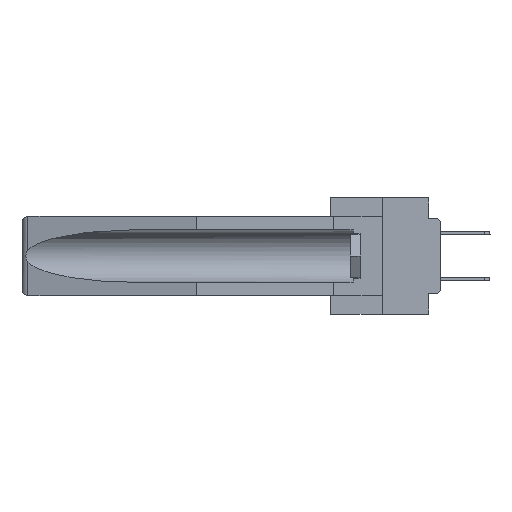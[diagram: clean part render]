
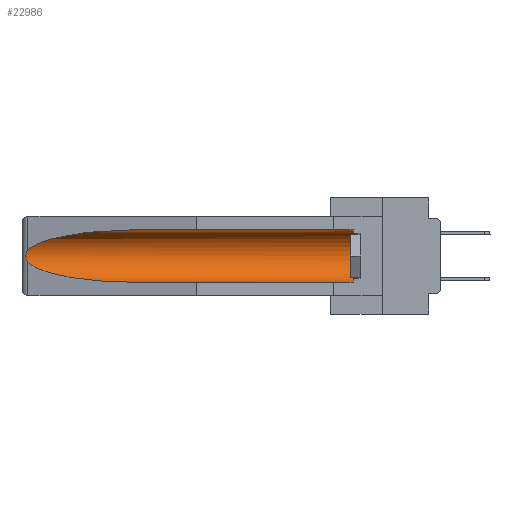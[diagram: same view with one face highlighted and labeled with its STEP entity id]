
A CAD part, left-side view. The second image highlights one B-rep face of the part: STEP entity #22986.
In plain terms, the highlighted cylindrical face has radius 2.857 mm (diameter 5.715 mm), a partial arc.
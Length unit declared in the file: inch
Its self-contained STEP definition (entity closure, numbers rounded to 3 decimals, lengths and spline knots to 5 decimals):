
#192 = CARTESIAN_POINT ( 'NONE',  ( 0.25451, 1.48313, -0.09465 ) ) ;
#2020 = FACE_OUTER_BOUND ( 'NONE', #16455, .T. ) ;
#2056 = ORIENTED_EDGE ( 'NONE', *, *, #12006, .T. ) ;
#2120 = CARTESIAN_POINT ( 'NONE',  ( 0.26537, 1.52718, -0.19328 ) ) ;
#2142 = CARTESIAN_POINT ( 'NONE',  ( 0.155, 1.07973, -0.284 ) ) ;
#2314 = CARTESIAN_POINT ( 'NONE',  ( 0.26537, 1.52718, -0.19328 ) ) ;
#2324 = CARTESIAN_POINT ( 'NONE',  ( 0.2673, 1.53269, -0.17917 ) ) ;
#2793 = EDGE_CURVE ( 'NONE', #16235, #20922, #7235, .T. ) ;
#2963 = EDGE_CURVE ( 'NONE', #4122, #29052, #12959, .T. ) ;
#3872 = CARTESIAN_POINT ( 'NONE',  ( 0.155, 1.07973, -0.059 ) ) ;
#4122 = VERTEX_POINT ( 'NONE', #9852 ) ;
#4868 = LINE ( 'NONE', #5699, #19625 ) ;
#5378 =( BOUNDED_CURVE ( )  B_SPLINE_CURVE ( 3, ( #25548, #13990, #192, #20624 ),
 .UNSPECIFIED., .F., .F. ) 
 B_SPLINE_CURVE_WITH_KNOTS ( ( 4, 4 ),
 ( 4.71239, 6.08839 ),
 .UNSPECIFIED. ) 
 CURVE ( )  GEOMETRIC_REPRESENTATION_ITEM ( )  RATIONAL_B_SPLINE_CURVE ( ( 1., 0.848, 0.848, 1. ) ) 
 REPRESENTATION_ITEM ( '' )  );
#5699 = CARTESIAN_POINT ( 'NONE',  ( 0.155, -0.30754, -0.284 ) ) ;
#5788 = VECTOR ( 'NONE', #6895, 39.37008 ) ;
#6256 = CARTESIAN_POINT ( 'NONE',  ( 0.26654, 1.53092, -0.15636 ) ) ;
#6895 = DIRECTION ( 'NONE',  ( 0., 1., 0. ) ) ;
#7235 =( BOUNDED_CURVE ( )  B_SPLINE_CURVE ( 3, ( #11639, #7424, #16296, #18592 ),
 .UNSPECIFIED., .F., .F. ) 
 B_SPLINE_CURVE_WITH_KNOTS ( ( 4, 4 ),
 ( 0.1948, 1.5708 ),
 .UNSPECIFIED. ) 
 CURVE ( )  GEOMETRIC_REPRESENTATION_ITEM ( )  RATIONAL_B_SPLINE_CURVE ( ( 1., 0.848, 0.848, 1. ) ) 
 REPRESENTATION_ITEM ( '' )  );
#7424 = CARTESIAN_POINT ( 'NONE',  ( 0.25451, 1.48313, -0.24835 ) ) ;
#8125 = CYLINDRICAL_SURFACE ( 'NONE', #21301, 0.1125 ) ;
#8450 = CARTESIAN_POINT ( 'NONE',  ( 0.26597, 1.52961, -0.15275 ) ) ;
#9852 = CARTESIAN_POINT ( 'NONE',  ( 0.155, 0.126, -0.059 ) ) ;
#10195 = DIRECTION ( 'NONE',  ( 0., 0., 1. ) ) ;
#10213 = DIRECTION ( 'NONE',  ( 0., 1., 0. ) ) ;
#10776 = CARTESIAN_POINT ( 'NONE',  ( 0.2675, 1.53308, -0.16763 ) ) ;
#11327 = VERTEX_POINT ( 'NONE', #21491 ) ;
#11628 = ORIENTED_EDGE ( 'NONE', *, *, #15197, .F. ) ;
#11639 = CARTESIAN_POINT ( 'NONE',  ( 0.26537, 1.52718, -0.19328 ) ) ;
#11834 = CARTESIAN_POINT ( 'NONE',  ( 0.155, -0.30754, -0.1715 ) ) ;
#12006 = EDGE_CURVE ( 'NONE', #11327, #4122, #24138, .T. ) ;
#12363 = EDGE_CURVE ( 'NONE', #29052, #29511, #5378, .T. ) ;
#12959 = LINE ( 'NONE', #14118, #5788 ) ;
#13074 = CARTESIAN_POINT ( 'NONE',  ( 0.2675, 1.53308, -0.17534 ) ) ;
#13815 = CARTESIAN_POINT ( 'NONE',  ( 0.26537, 1.52718, -0.14972 ) ) ;
#13990 = CARTESIAN_POINT ( 'NONE',  ( 0.21114, 1.30732, -0.059 ) ) ;
#14118 = CARTESIAN_POINT ( 'NONE',  ( 0.155, -0.30754, -0.059 ) ) ;
#14432 = B_SPLINE_CURVE_WITH_KNOTS ( 'NONE', 3,
 ( #18319, #8450, #6256, #24533, #10776, #13074, #2324, #29193, #15297, #2120 ),
 .UNSPECIFIED., .F., .F.,
 ( 4, 2, 2, 2, 4 ),
 ( 0., 0.00029, 0.00058, 0.00087, 0.00117 ),
 .UNSPECIFIED. ) ;
#15197 = EDGE_CURVE ( 'NONE', #11327, #20922, #4868, .T. ) ;
#15297 = CARTESIAN_POINT ( 'NONE',  ( 0.26597, 1.5296, -0.19026 ) ) ;
#16235 = VERTEX_POINT ( 'NONE', #2314 ) ;
#16296 = CARTESIAN_POINT ( 'NONE',  ( 0.21114, 1.30732, -0.284 ) ) ;
#16455 = EDGE_LOOP ( 'NONE', ( #20876, #25119, #20142, #11628, #2056, #27660 ) ) ;
#18319 = CARTESIAN_POINT ( 'NONE',  ( 0.26537, 1.52718, -0.14972 ) ) ;
#18592 = CARTESIAN_POINT ( 'NONE',  ( 0.155, 1.07973, -0.284 ) ) ;
#19348 = CARTESIAN_POINT ( 'NONE',  ( 0.155, 0.126, -0.1715 ) ) ;
#19625 = VECTOR ( 'NONE', #10213, 39.37008 ) ;
#20142 = ORIENTED_EDGE ( 'NONE', *, *, #2793, .T. ) ;
#20624 = CARTESIAN_POINT ( 'NONE',  ( 0.26537, 1.52718, -0.14972 ) ) ;
#20876 = ORIENTED_EDGE ( 'NONE', *, *, #12363, .T. ) ;
#20922 = VERTEX_POINT ( 'NONE', #2142 ) ;
#21301 = AXIS2_PLACEMENT_3D ( 'NONE', #11834, #25324, #23384 ) ;
#21491 = CARTESIAN_POINT ( 'NONE',  ( 0.155, 0.126, -0.284 ) ) ;
#22986 = ADVANCED_FACE ( 'NONE', ( #2020 ), #8125, .F. ) ;
#23384 = DIRECTION ( 'NONE',  ( 0., 0., 1. ) ) ;
#24138 = CIRCLE ( 'NONE', #27842, 0.1125 ) ;
#24533 = CARTESIAN_POINT ( 'NONE',  ( 0.2673, 1.5327, -0.16383 ) ) ;
#25119 = ORIENTED_EDGE ( 'NONE', *, *, #25234, .T. ) ;
#25234 = EDGE_CURVE ( 'NONE', #29511, #16235, #14432, .T. ) ;
#25324 = DIRECTION ( 'NONE',  ( 0., 1., 0. ) ) ;
#25548 = CARTESIAN_POINT ( 'NONE',  ( 0.155, 1.07973, -0.059 ) ) ;
#26000 = DIRECTION ( 'NONE',  ( 0., -1., 0. ) ) ;
#27660 = ORIENTED_EDGE ( 'NONE', *, *, #2963, .T. ) ;
#27842 = AXIS2_PLACEMENT_3D ( 'NONE', #19348, #26000, #10195 ) ;
#29052 = VERTEX_POINT ( 'NONE', #3872 ) ;
#29193 = CARTESIAN_POINT ( 'NONE',  ( 0.26655, 1.53094, -0.18657 ) ) ;
#29511 = VERTEX_POINT ( 'NONE', #13815 ) ;
